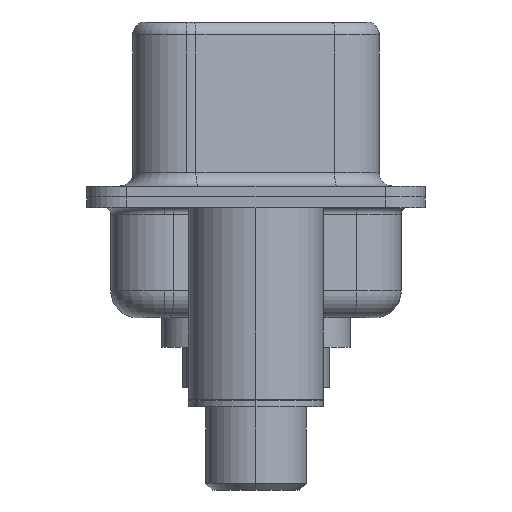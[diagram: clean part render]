
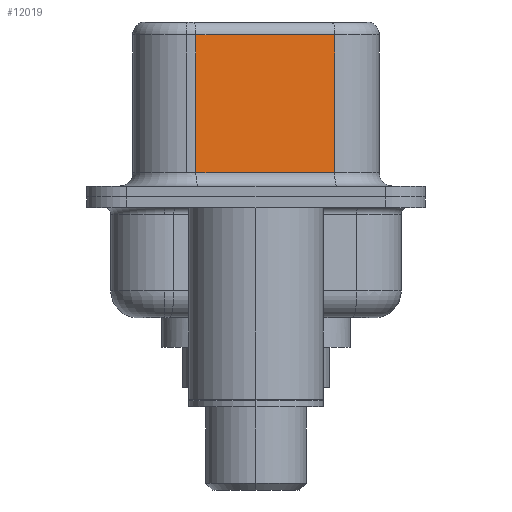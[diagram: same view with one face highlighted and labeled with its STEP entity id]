
A CAD part, left-side view. The second image highlights one B-rep face of the part: STEP entity #12019.
In plain terms, the highlighted planar face has unit normal (-0.985, -0.174, 0).
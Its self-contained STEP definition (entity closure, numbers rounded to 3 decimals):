
#60 = DIRECTION ( 'NONE',  ( 0.985, 0.174, 0. ) ) ;
#1063 = LINE ( 'NONE', #7121, #10355 ) ;
#1574 = AXIS2_PLACEMENT_3D ( 'NONE', #6973, #60, #8148 ) ;
#2405 = CARTESIAN_POINT ( 'NONE',  ( 4.585, -2.927, 6.02 ) ) ;
#2575 = VECTOR ( 'NONE', #11883, 1000. ) ;
#2858 = VERTEX_POINT ( 'NONE', #14754 ) ;
#3559 = DIRECTION ( 'NONE',  ( 0.174, -0.985, 0. ) ) ;
#3632 = EDGE_LOOP ( 'NONE', ( #8773, #5531, #6924, #6453 ) ) ;
#3702 = EDGE_CURVE ( 'NONE', #6386, #2858, #11864, .T. ) ;
#3810 = EDGE_CURVE ( 'NONE', #2858, #9673, #13894, .T. ) ;
#3901 = VECTOR ( 'NONE', #3559, 1000. ) ;
#4151 = CARTESIAN_POINT ( 'NONE',  ( 3.675, 2.233, 0.9 ) ) ;
#4364 = CARTESIAN_POINT ( 'NONE',  ( 4.585, -2.927, 0.9 ) ) ;
#5531 = ORIENTED_EDGE ( 'NONE', *, *, #3702, .T. ) ;
#5822 = PLANE ( 'NONE',  #1574 ) ;
#6006 = DIRECTION ( 'NONE',  ( 0., 0., -1. ) ) ;
#6052 = CARTESIAN_POINT ( 'NONE',  ( 3.675, 2.233, 6.52 ) ) ;
#6386 = VERTEX_POINT ( 'NONE', #2405 ) ;
#6453 = ORIENTED_EDGE ( 'NONE', *, *, #8332, .T. ) ;
#6462 = CARTESIAN_POINT ( 'NONE',  ( 4.585, -2.927, 0.9 ) ) ;
#6586 = EDGE_CURVE ( 'NONE', #6386, #7680, #1063, .T. ) ;
#6924 = ORIENTED_EDGE ( 'NONE', *, *, #3810, .T. ) ;
#6973 = CARTESIAN_POINT ( 'NONE',  ( 4.585, -2.927, 6.52 ) ) ;
#7121 = CARTESIAN_POINT ( 'NONE',  ( 4.585, -2.927, 6.52 ) ) ;
#7459 = DIRECTION ( 'NONE',  ( 0., 0., -1. ) ) ;
#7674 = VECTOR ( 'NONE', #6006, 1000. ) ;
#7680 = VERTEX_POINT ( 'NONE', #6462 ) ;
#8148 = DIRECTION ( 'NONE',  ( -0.174, 0.985, 0. ) ) ;
#8332 = EDGE_CURVE ( 'NONE', #9673, #7680, #10481, .T. ) ;
#8465 = FACE_OUTER_BOUND ( 'NONE', #3632, .T. ) ;
#8773 = ORIENTED_EDGE ( 'NONE', *, *, #6586, .F. ) ;
#9673 = VERTEX_POINT ( 'NONE', #4151 ) ;
#10355 = VECTOR ( 'NONE', #7459, 1000. ) ;
#10481 = LINE ( 'NONE', #4364, #3901 ) ;
#11839 = CARTESIAN_POINT ( 'NONE',  ( 4.585, -2.927, 6.02 ) ) ;
#11864 = LINE ( 'NONE', #11839, #2575 ) ;
#11883 = DIRECTION ( 'NONE',  ( -0.174, 0.985, 0. ) ) ;
#12019 = ADVANCED_FACE ( 'NONE', ( #8465 ), #5822, .F. ) ;
#13894 = LINE ( 'NONE', #6052, #7674 ) ;
#14754 = CARTESIAN_POINT ( 'NONE',  ( 3.675, 2.233, 6.02 ) ) ;
